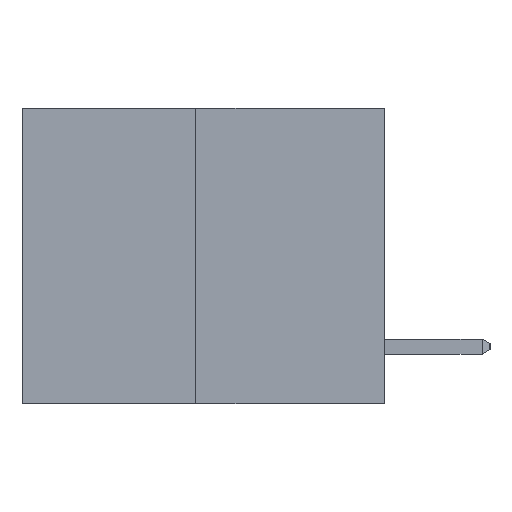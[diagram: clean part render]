
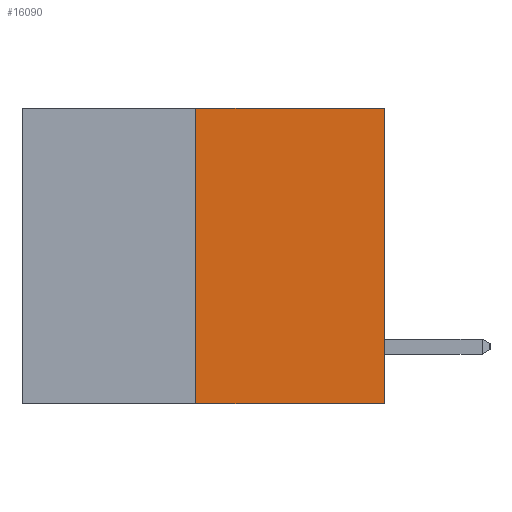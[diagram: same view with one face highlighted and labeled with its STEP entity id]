
A CAD part, left-side view. The second image highlights one B-rep face of the part: STEP entity #16090.
In plain terms, the highlighted planar face has unit normal (-1, 0, 0).
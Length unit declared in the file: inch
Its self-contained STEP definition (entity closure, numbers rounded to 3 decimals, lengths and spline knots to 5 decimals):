
#1058 = ORIENTED_EDGE ( 'NONE', *, *, #10603, .F. ) ;
#1561 = DIRECTION ( 'NONE',  ( 0., -1., 0. ) ) ;
#3387 = VECTOR ( 'NONE', #14310, 39.37008 ) ;
#3908 = ORIENTED_EDGE ( 'NONE', *, *, #16799, .T. ) ;
#4774 = VERTEX_POINT ( 'NONE', #17885 ) ;
#4941 = VERTEX_POINT ( 'NONE', #8908 ) ;
#5188 = VERTEX_POINT ( 'NONE', #8783 ) ;
#5832 = LINE ( 'NONE', #18382, #22698 ) ;
#5938 = DIRECTION ( 'NONE',  ( 0., 0., -1. ) ) ;
#6786 = AXIS2_PLACEMENT_3D ( 'NONE', #11297, #11053, #5938 ) ;
#7021 = PLANE ( 'NONE',  #6786 ) ;
#8783 = CARTESIAN_POINT ( 'NONE',  ( 0., 0.312, 0. ) ) ;
#8908 = CARTESIAN_POINT ( 'NONE',  ( 0., 0.312, -0.49 ) ) ;
#9351 = CARTESIAN_POINT ( 'NONE',  ( 0., 0., 0. ) ) ;
#10593 = VERTEX_POINT ( 'NONE', #9351 ) ;
#10603 = EDGE_CURVE ( 'NONE', #5188, #10593, #20907, .T. ) ;
#11053 = DIRECTION ( 'NONE',  ( 1., 0., 0. ) ) ;
#11297 = CARTESIAN_POINT ( 'NONE',  ( 0., 0.6, 0. ) ) ;
#12400 = CARTESIAN_POINT ( 'NONE',  ( 0., 0.312, -0.49 ) ) ;
#12954 = DIRECTION ( 'NONE',  ( 0., -1., 0. ) ) ;
#12995 = EDGE_LOOP ( 'NONE', ( #13155, #21782, #3908, #1058 ) ) ;
#13155 = ORIENTED_EDGE ( 'NONE', *, *, #22359, .F. ) ;
#14310 = DIRECTION ( 'NONE',  ( 0., 0., 1. ) ) ;
#14966 = EDGE_CURVE ( 'NONE', #4941, #4774, #15422, .T. ) ;
#15099 = VECTOR ( 'NONE', #12954, 39.37008 ) ;
#15422 = LINE ( 'NONE', #20336, #15099 ) ;
#16090 = ADVANCED_FACE ( 'NONE', ( #22659 ), #7021, .F. ) ;
#16488 = DIRECTION ( 'NONE',  ( 0., 0., 1. ) ) ;
#16799 = EDGE_CURVE ( 'NONE', #4774, #10593, #5832, .T. ) ;
#16838 = CARTESIAN_POINT ( 'NONE',  ( 0., 0.6, 0. ) ) ;
#17885 = CARTESIAN_POINT ( 'NONE',  ( 0., 0., -0.49 ) ) ;
#18382 = CARTESIAN_POINT ( 'NONE',  ( 0., 0., 0. ) ) ;
#19724 = VECTOR ( 'NONE', #1561, 39.37008 ) ;
#20336 = CARTESIAN_POINT ( 'NONE',  ( 0., 0.6, -0.49 ) ) ;
#20907 = LINE ( 'NONE', #16838, #19724 ) ;
#21782 = ORIENTED_EDGE ( 'NONE', *, *, #14966, .T. ) ;
#22359 = EDGE_CURVE ( 'NONE', #4941, #5188, #24093, .T. ) ;
#22659 = FACE_OUTER_BOUND ( 'NONE', #12995, .T. ) ;
#22698 = VECTOR ( 'NONE', #16488, 39.37008 ) ;
#24093 = LINE ( 'NONE', #12400, #3387 ) ;
